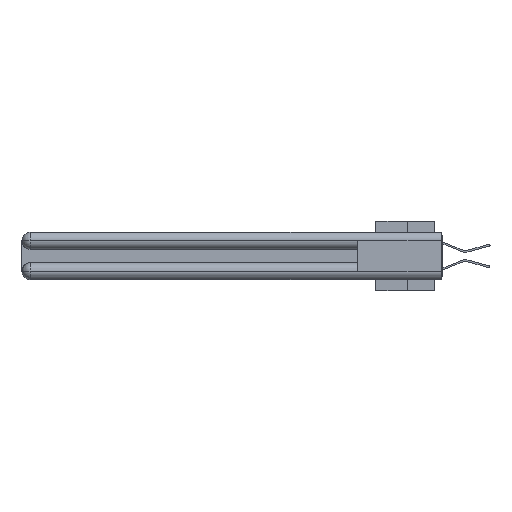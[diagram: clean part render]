
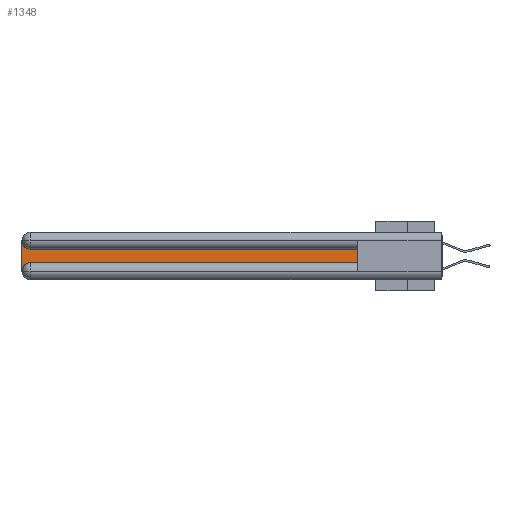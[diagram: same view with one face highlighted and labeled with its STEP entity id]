
A CAD part, left-side view. The second image highlights one B-rep face of the part: STEP entity #1348.
In plain terms, the highlighted planar face has unit normal (-1, 0, 0).
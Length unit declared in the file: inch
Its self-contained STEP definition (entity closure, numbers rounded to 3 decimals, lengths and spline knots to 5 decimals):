
#1348 = ADVANCED_FACE ( 'NONE', ( #17972 ), #32328, .F. ) ;
#1485 = DIRECTION ( 'NONE',  ( 0., 0., 1. ) ) ;
#1865 = CARTESIAN_POINT ( 'NONE',  ( 0.075, 0.6, -0.1225 ) ) ;
#2511 = DIRECTION ( 'NONE',  ( 1., 0., 0. ) ) ;
#2610 = VERTEX_POINT ( 'NONE', #22804 ) ;
#2899 = LINE ( 'NONE', #13833, #25056 ) ;
#3822 = CARTESIAN_POINT ( 'NONE',  ( 0.075, 0.6, -0.1225 ) ) ;
#4000 = LINE ( 'NONE', #3822, #37749 ) ;
#4194 = EDGE_CURVE ( 'NONE', #19271, #2610, #2899, .T. ) ;
#6206 = CARTESIAN_POINT ( 'NONE',  ( 0.075, 2.94, -0.1225 ) ) ;
#6694 = DIRECTION ( 'NONE',  ( 0., 1., 0. ) ) ;
#8273 = ORIENTED_EDGE ( 'NONE', *, *, #8379, .T. ) ;
#8379 = EDGE_CURVE ( 'NONE', #2610, #8655, #16770, .T. ) ;
#8655 = VERTEX_POINT ( 'NONE', #13103 ) ;
#10183 = AXIS2_PLACEMENT_3D ( 'NONE', #14381, #2511, #16496 ) ;
#12145 = EDGE_CURVE ( 'NONE', #36983, #19271, #20551, .T. ) ;
#12602 = LINE ( 'NONE', #36498, #28013 ) ;
#13103 = CARTESIAN_POINT ( 'NONE',  ( 0.075, 2.94, -0.2175 ) ) ;
#13833 = CARTESIAN_POINT ( 'NONE',  ( 0.075, 3., -0.2175 ) ) ;
#14016 = EDGE_CURVE ( 'NONE', #18056, #16553, #12602, .T. ) ;
#14128 = ORIENTED_EDGE ( 'NONE', *, *, #4194, .T. ) ;
#14381 = CARTESIAN_POINT ( 'NONE',  ( 0.075, 2.94, -0.0625 ) ) ;
#14658 = ORIENTED_EDGE ( 'NONE', *, *, #18901, .T. ) ;
#16136 = AXIS2_PLACEMENT_3D ( 'NONE', #35576, #26575, #23321 ) ;
#16496 = DIRECTION ( 'NONE',  ( 0., 0., -1. ) ) ;
#16553 = VERTEX_POINT ( 'NONE', #1865 ) ;
#16770 = CIRCLE ( 'NONE', #37537, 0.06 ) ;
#17972 = FACE_OUTER_BOUND ( 'NONE', #20950, .T. ) ;
#18014 = DIRECTION ( 'NONE',  ( 0., -1., 0. ) ) ;
#18056 = VERTEX_POINT ( 'NONE', #35363 ) ;
#18901 = EDGE_CURVE ( 'NONE', #16553, #36983, #4000, .T. ) ;
#19271 = VERTEX_POINT ( 'NONE', #28861 ) ;
#19946 = DIRECTION ( 'NONE',  ( 0., 0., -1. ) ) ;
#20336 = VECTOR ( 'NONE', #18014, 39.37008 ) ;
#20551 = CIRCLE ( 'NONE', #10183, 0.06 ) ;
#20680 = LINE ( 'NONE', #35979, #20336 ) ;
#20950 = EDGE_LOOP ( 'NONE', ( #14658, #36189, #14128, #8273, #24695, #22503 ) ) ;
#22141 = CARTESIAN_POINT ( 'NONE',  ( 0.075, 2.94, -0.2775 ) ) ;
#22503 = ORIENTED_EDGE ( 'NONE', *, *, #14016, .T. ) ;
#22804 = CARTESIAN_POINT ( 'NONE',  ( 0.075, 3., -0.2775 ) ) ;
#23321 = DIRECTION ( 'NONE',  ( 0., 0., -1. ) ) ;
#24695 = ORIENTED_EDGE ( 'NONE', *, *, #25674, .T. ) ;
#25056 = VECTOR ( 'NONE', #19946, 39.37008 ) ;
#25674 = EDGE_CURVE ( 'NONE', #8655, #18056, #20680, .T. ) ;
#26575 = DIRECTION ( 'NONE',  ( 1., 0., 0. ) ) ;
#28013 = VECTOR ( 'NONE', #1485, 39.37008 ) ;
#28861 = CARTESIAN_POINT ( 'NONE',  ( 0.075, 3., -0.0625 ) ) ;
#29394 = DIRECTION ( 'NONE',  ( 0., 0., -1. ) ) ;
#32277 = DIRECTION ( 'NONE',  ( 1., 0., 0. ) ) ;
#32328 = PLANE ( 'NONE',  #16136 ) ;
#35363 = CARTESIAN_POINT ( 'NONE',  ( 0.075, 0.6, -0.2175 ) ) ;
#35576 = CARTESIAN_POINT ( 'NONE',  ( 0.075, 3., -0.1225 ) ) ;
#35979 = CARTESIAN_POINT ( 'NONE',  ( 0.075, 0.6, -0.2175 ) ) ;
#36189 = ORIENTED_EDGE ( 'NONE', *, *, #12145, .T. ) ;
#36498 = CARTESIAN_POINT ( 'NONE',  ( 0.075, 0.6, -0.2175 ) ) ;
#36983 = VERTEX_POINT ( 'NONE', #6206 ) ;
#37537 = AXIS2_PLACEMENT_3D ( 'NONE', #22141, #32277, #29394 ) ;
#37749 = VECTOR ( 'NONE', #6694, 39.37008 ) ;
